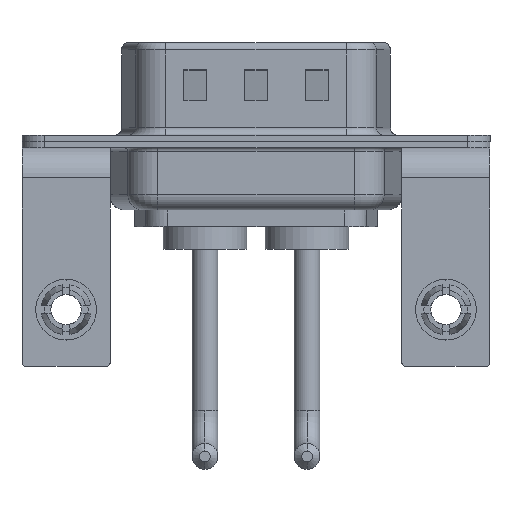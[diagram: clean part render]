
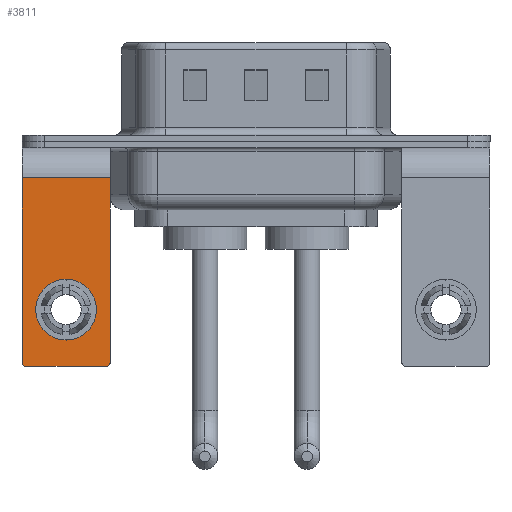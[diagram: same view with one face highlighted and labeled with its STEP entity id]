
A CAD part, front view. The second image highlights one B-rep face of the part: STEP entity #3811.
In plain terms, the highlighted planar face has unit normal (0, -1, 0).
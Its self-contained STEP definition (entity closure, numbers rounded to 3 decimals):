
#51 = ORIENTED_EDGE ( 'NONE', *, *, #8893, .F. ) ;
#161 = CARTESIAN_POINT ( 'NONE',  ( 2.9, -6.25, -2.4 ) ) ;
#684 = CARTESIAN_POINT ( 'NONE',  ( -2.9, -6.25, -2.4 ) ) ;
#928 = AXIS2_PLACEMENT_3D ( 'NONE', #14223, #1503, #11690 ) ;
#1023 = EDGE_CURVE ( 'NONE', #13738, #16466, #8671, .T. ) ;
#1039 = EDGE_LOOP ( 'NONE', ( #1256, #15304, #51, #15108, #8882, #10120 ) ) ;
#1042 = EDGE_CURVE ( 'NONE', #2481, #2493, #5694, .T. ) ;
#1256 = ORIENTED_EDGE ( 'NONE', *, *, #8192, .T. ) ;
#1503 = DIRECTION ( 'NONE',  ( 0., 1., 0. ) ) ;
#1758 = EDGE_LOOP ( 'NONE', ( #9446, #7943 ) ) ;
#1932 = CARTESIAN_POINT ( 'NONE',  ( 2.9, -6.25, -2.4 ) ) ;
#2030 = DIRECTION ( 'NONE',  ( 0., 0., 1. ) ) ;
#2247 = CARTESIAN_POINT ( 'NONE',  ( 2.9, -6.25, -14.8 ) ) ;
#2481 = VERTEX_POINT ( 'NONE', #8804 ) ;
#2493 = VERTEX_POINT ( 'NONE', #13964 ) ;
#2776 = DIRECTION ( 'NONE',  ( 0., 0., -1. ) ) ;
#3120 = CARTESIAN_POINT ( 'NONE',  ( 2.9, -6.25, -14.55 ) ) ;
#3537 = CARTESIAN_POINT ( 'NONE',  ( -2.9, -6.25, -14.55 ) ) ;
#3811 = ADVANCED_FACE ( 'NONE', ( #6522, #9056 ), #7713, .F. ) ;
#3923 = EDGE_CURVE ( 'NONE', #4523, #16466, #15900, .T. ) ;
#4410 = CIRCLE ( 'NONE', #9283, 0.25 ) ;
#4523 = VERTEX_POINT ( 'NONE', #161 ) ;
#5669 = AXIS2_PLACEMENT_3D ( 'NONE', #7683, #10311, #12691 ) ;
#5694 = CIRCLE ( 'NONE', #16517, 2. ) ;
#6071 = LINE ( 'NONE', #2247, #13099 ) ;
#6522 = FACE_BOUND ( 'NONE', #1758, .T. ) ;
#6593 = VECTOR ( 'NONE', #2776, 1000. ) ;
#6805 = CARTESIAN_POINT ( 'NONE',  ( 2.65, -6.25, -14.8 ) ) ;
#7029 = CARTESIAN_POINT ( 'NONE',  ( -2.65, -6.25, -14.55 ) ) ;
#7101 = DIRECTION ( 'NONE',  ( 0., 0., -1. ) ) ;
#7683 = CARTESIAN_POINT ( 'NONE',  ( 0., -6.25, -11.07 ) ) ;
#7713 = PLANE ( 'NONE',  #928 ) ;
#7769 = EDGE_CURVE ( 'NONE', #10868, #8104, #4410, .T. ) ;
#7820 = LINE ( 'NONE', #12992, #14244 ) ;
#7943 = ORIENTED_EDGE ( 'NONE', *, *, #1042, .T. ) ;
#8023 = CARTESIAN_POINT ( 'NONE',  ( -2.9, -6.25, -2.4 ) ) ;
#8104 = VERTEX_POINT ( 'NONE', #12708 ) ;
#8192 = EDGE_CURVE ( 'NONE', #15884, #10868, #14376, .T. ) ;
#8671 = CIRCLE ( 'NONE', #13277, 0.25 ) ;
#8804 = CARTESIAN_POINT ( 'NONE',  ( 0., -6.25, -9.07 ) ) ;
#8882 = ORIENTED_EDGE ( 'NONE', *, *, #3923, .F. ) ;
#8893 = EDGE_CURVE ( 'NONE', #13738, #8104, #6071, .T. ) ;
#9056 = FACE_OUTER_BOUND ( 'NONE', #1039, .T. ) ;
#9283 = AXIS2_PLACEMENT_3D ( 'NONE', #7029, #13395, #10854 ) ;
#9446 = ORIENTED_EDGE ( 'NONE', *, *, #14478, .T. ) ;
#9739 = DIRECTION ( 'NONE',  ( 0., 1., 0. ) ) ;
#9813 = EDGE_CURVE ( 'NONE', #4523, #15884, #7820, .T. ) ;
#10120 = ORIENTED_EDGE ( 'NONE', *, *, #9813, .T. ) ;
#10311 = DIRECTION ( 'NONE',  ( 0., 1., 0. ) ) ;
#10854 = DIRECTION ( 'NONE',  ( 0., 0., 1. ) ) ;
#10868 = VERTEX_POINT ( 'NONE', #3537 ) ;
#11669 = CIRCLE ( 'NONE', #5669, 2. ) ;
#11690 = DIRECTION ( 'NONE',  ( 0., 0., 1. ) ) ;
#11734 = DIRECTION ( 'NONE',  ( -1., 0., 0. ) ) ;
#12455 = CARTESIAN_POINT ( 'NONE',  ( 0., -6.25, -11.07 ) ) ;
#12544 = CARTESIAN_POINT ( 'NONE',  ( 2.65, -6.25, -14.55 ) ) ;
#12673 = DIRECTION ( 'NONE',  ( -1., 0., 0. ) ) ;
#12691 = DIRECTION ( 'NONE',  ( 0., 0., 1. ) ) ;
#12708 = CARTESIAN_POINT ( 'NONE',  ( -2.65, -6.25, -14.8 ) ) ;
#12992 = CARTESIAN_POINT ( 'NONE',  ( 2.9, -6.25, -2.4 ) ) ;
#13014 = VECTOR ( 'NONE', #7101, 1000. ) ;
#13099 = VECTOR ( 'NONE', #12673, 1000. ) ;
#13277 = AXIS2_PLACEMENT_3D ( 'NONE', #12544, #13803, #2030 ) ;
#13395 = DIRECTION ( 'NONE',  ( 0., -1., 0. ) ) ;
#13738 = VERTEX_POINT ( 'NONE', #6805 ) ;
#13803 = DIRECTION ( 'NONE',  ( 0., -1., 0. ) ) ;
#13964 = CARTESIAN_POINT ( 'NONE',  ( 0., -6.25, -13.07 ) ) ;
#14223 = CARTESIAN_POINT ( 'NONE',  ( 2.9, -6.25, -2.4 ) ) ;
#14244 = VECTOR ( 'NONE', #11734, 1000. ) ;
#14376 = LINE ( 'NONE', #8023, #6593 ) ;
#14478 = EDGE_CURVE ( 'NONE', #2493, #2481, #11669, .T. ) ;
#14901 = DIRECTION ( 'NONE',  ( 0., 0., 1. ) ) ;
#15108 = ORIENTED_EDGE ( 'NONE', *, *, #1023, .T. ) ;
#15304 = ORIENTED_EDGE ( 'NONE', *, *, #7769, .T. ) ;
#15884 = VERTEX_POINT ( 'NONE', #684 ) ;
#15900 = LINE ( 'NONE', #1932, #13014 ) ;
#16466 = VERTEX_POINT ( 'NONE', #3120 ) ;
#16517 = AXIS2_PLACEMENT_3D ( 'NONE', #12455, #9739, #14901 ) ;
